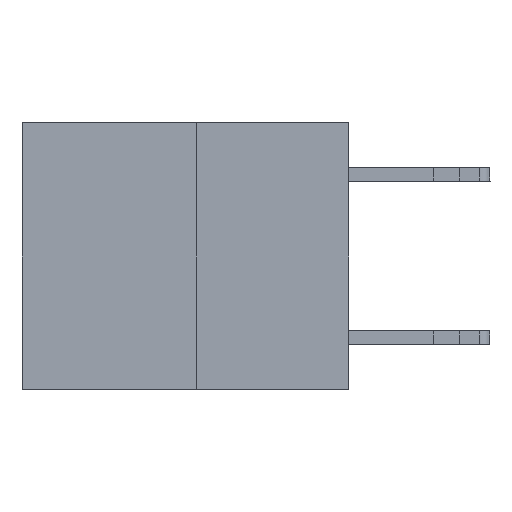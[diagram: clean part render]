
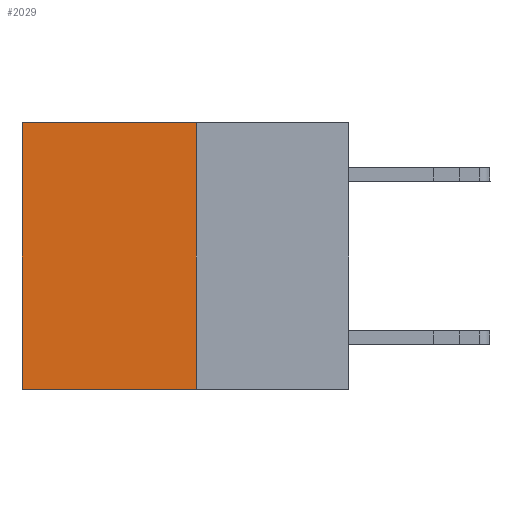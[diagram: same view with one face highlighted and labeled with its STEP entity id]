
A CAD part, left-side view. The second image highlights one B-rep face of the part: STEP entity #2029.
In plain terms, the highlighted planar face has unit normal (-1, 0, 0).
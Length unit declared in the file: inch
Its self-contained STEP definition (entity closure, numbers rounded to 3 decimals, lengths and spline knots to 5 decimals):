
#10 = DIRECTION ( 'NONE',  ( 0., 1., 0. ) ) ;
#462 = CARTESIAN_POINT ( 'NONE',  ( 0.3165, 0.6, 0. ) ) ;
#1175 = LINE ( 'NONE', #15673, #19687 ) ;
#1452 = VECTOR ( 'NONE', #18843, 39.37008 ) ;
#1851 = CARTESIAN_POINT ( 'NONE',  ( 0.3165, 0.6, -0.49 ) ) ;
#1961 = VECTOR ( 'NONE', #6314, 39.37008 ) ;
#2029 = ADVANCED_FACE ( 'NONE', ( #15890 ), #2506, .F. ) ;
#2082 = EDGE_LOOP ( 'NONE', ( #23868, #22985, #16615, #2337 ) ) ;
#2337 = ORIENTED_EDGE ( 'NONE', *, *, #22261, .T. ) ;
#2506 = PLANE ( 'NONE',  #11769 ) ;
#4290 = VERTEX_POINT ( 'NONE', #16563 ) ;
#5485 = DIRECTION ( 'NONE',  ( 0., 0., -1. ) ) ;
#6008 = CARTESIAN_POINT ( 'NONE',  ( 0.3165, 0.28, -0.49 ) ) ;
#6314 = DIRECTION ( 'NONE',  ( 0., 0., -1. ) ) ;
#7840 = DIRECTION ( 'NONE',  ( 1., 0., 0. ) ) ;
#8781 = VERTEX_POINT ( 'NONE', #10379 ) ;
#9256 = LINE ( 'NONE', #13376, #1452 ) ;
#10379 = CARTESIAN_POINT ( 'NONE',  ( 0.3165, 0.28, -0.49 ) ) ;
#11769 = AXIS2_PLACEMENT_3D ( 'NONE', #6008, #7840, #5485 ) ;
#12119 = CARTESIAN_POINT ( 'NONE',  ( 0.3165, 0.6, -0.49 ) ) ;
#13376 = CARTESIAN_POINT ( 'NONE',  ( 0.3165, 0.28, 0. ) ) ;
#13746 = DIRECTION ( 'NONE',  ( 0., 0., -1. ) ) ;
#14427 = LINE ( 'NONE', #12119, #1961 ) ;
#14986 = VERTEX_POINT ( 'NONE', #462 ) ;
#15068 = CARTESIAN_POINT ( 'NONE',  ( 0.3165, 0.28, -0.49 ) ) ;
#15673 = CARTESIAN_POINT ( 'NONE',  ( 0.3165, 0.28, -0.49 ) ) ;
#15890 = FACE_OUTER_BOUND ( 'NONE', #2082, .T. ) ;
#16563 = CARTESIAN_POINT ( 'NONE',  ( 0.3165, 0.28, 0. ) ) ;
#16615 = ORIENTED_EDGE ( 'NONE', *, *, #21202, .F. ) ;
#17008 = LINE ( 'NONE', #15068, #17303 ) ;
#17303 = VECTOR ( 'NONE', #10, 39.37008 ) ;
#18843 = DIRECTION ( 'NONE',  ( 0., 1., 0. ) ) ;
#19687 = VECTOR ( 'NONE', #13746, 39.37008 ) ;
#21202 = EDGE_CURVE ( 'NONE', #4290, #8781, #1175, .T. ) ;
#22261 = EDGE_CURVE ( 'NONE', #4290, #14986, #9256, .T. ) ;
#22985 = ORIENTED_EDGE ( 'NONE', *, *, #23775, .F. ) ;
#23455 = VERTEX_POINT ( 'NONE', #1851 ) ;
#23585 = EDGE_CURVE ( 'NONE', #14986, #23455, #14427, .T. ) ;
#23775 = EDGE_CURVE ( 'NONE', #8781, #23455, #17008, .T. ) ;
#23868 = ORIENTED_EDGE ( 'NONE', *, *, #23585, .T. ) ;
